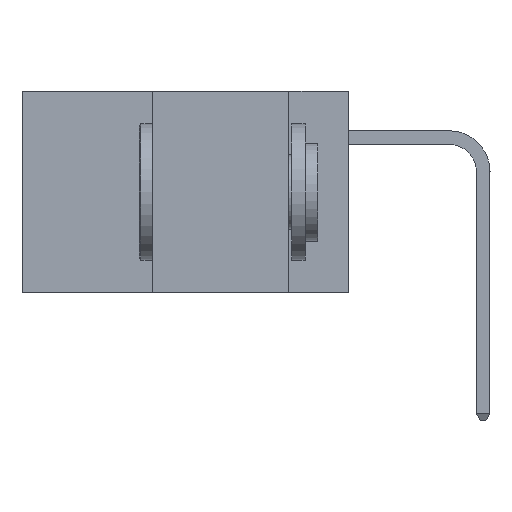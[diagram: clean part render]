
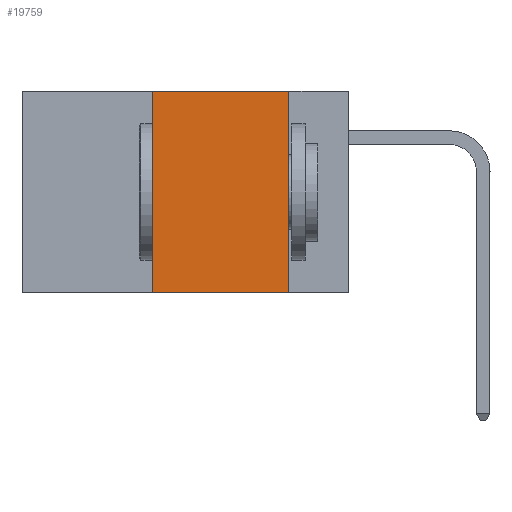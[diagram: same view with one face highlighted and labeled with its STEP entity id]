
A CAD part, left-side view. The second image highlights one B-rep face of the part: STEP entity #19759.
In plain terms, the highlighted planar face has unit normal (-1, 0, 0).
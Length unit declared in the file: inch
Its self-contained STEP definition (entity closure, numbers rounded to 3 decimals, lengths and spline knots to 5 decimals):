
#498 = VERTEX_POINT ( 'NONE', #43572 ) ;
#1414 = VERTEX_POINT ( 'NONE', #6823 ) ;
#1972 = ORIENTED_EDGE ( 'NONE', *, *, #42609, .F. ) ;
#4373 = CARTESIAN_POINT ( 'NONE',  ( 0., 0.36, 0. ) ) ;
#6347 = LINE ( 'NONE', #29264, #45518 ) ;
#6823 = CARTESIAN_POINT ( 'NONE',  ( 0., 0.11, -0.37 ) ) ;
#9359 = ORIENTED_EDGE ( 'NONE', *, *, #27717, .F. ) ;
#9562 = PLANE ( 'NONE',  #25301 ) ;
#10264 = VECTOR ( 'NONE', #27301, 39.37008 ) ;
#13045 = CARTESIAN_POINT ( 'NONE',  ( 0., 0.36, 0. ) ) ;
#13158 = VECTOR ( 'NONE', #38589, 39.37008 ) ;
#13444 = DIRECTION ( 'NONE',  ( 1., 0., 0. ) ) ;
#13756 = EDGE_CURVE ( 'NONE', #498, #1414, #23378, .T. ) ;
#13936 = VERTEX_POINT ( 'NONE', #13045 ) ;
#16433 = CARTESIAN_POINT ( 'NONE',  ( 0., 0.6, 0. ) ) ;
#19759 = ADVANCED_FACE ( 'NONE', ( #41450 ), #9562, .F. ) ;
#20532 = LINE ( 'NONE', #4373, #10264 ) ;
#21528 = EDGE_LOOP ( 'NONE', ( #1972, #9359, #44463, #43344 ) ) ;
#22042 = VERTEX_POINT ( 'NONE', #25826 ) ;
#23145 = LINE ( 'NONE', #16433, #43135 ) ;
#23378 = LINE ( 'NONE', #38429, #13158 ) ;
#25301 = AXIS2_PLACEMENT_3D ( 'NONE', #36156, #13444, #39946 ) ;
#25826 = CARTESIAN_POINT ( 'NONE',  ( 0., 0.11, 0. ) ) ;
#27301 = DIRECTION ( 'NONE',  ( 0., 0., 1. ) ) ;
#27717 = EDGE_CURVE ( 'NONE', #13936, #22042, #23145, .T. ) ;
#27747 = DIRECTION ( 'NONE',  ( 0., -1., 0. ) ) ;
#29264 = CARTESIAN_POINT ( 'NONE',  ( 0., 0.11, 0. ) ) ;
#36156 = CARTESIAN_POINT ( 'NONE',  ( 0., 0.6, 0. ) ) ;
#38429 = CARTESIAN_POINT ( 'NONE',  ( 0., 0.6, -0.37 ) ) ;
#38589 = DIRECTION ( 'NONE',  ( 0., -1., 0. ) ) ;
#39946 = DIRECTION ( 'NONE',  ( 0., 0., -1. ) ) ;
#41450 = FACE_OUTER_BOUND ( 'NONE', #21528, .T. ) ;
#42609 = EDGE_CURVE ( 'NONE', #22042, #1414, #6347, .T. ) ;
#43135 = VECTOR ( 'NONE', #27747, 39.37008 ) ;
#43344 = ORIENTED_EDGE ( 'NONE', *, *, #13756, .T. ) ;
#43572 = CARTESIAN_POINT ( 'NONE',  ( 0., 0.36, -0.37 ) ) ;
#44364 = DIRECTION ( 'NONE',  ( 0., 0., -1. ) ) ;
#44463 = ORIENTED_EDGE ( 'NONE', *, *, #47630, .F. ) ;
#45518 = VECTOR ( 'NONE', #44364, 39.37008 ) ;
#47630 = EDGE_CURVE ( 'NONE', #498, #13936, #20532, .T. ) ;
